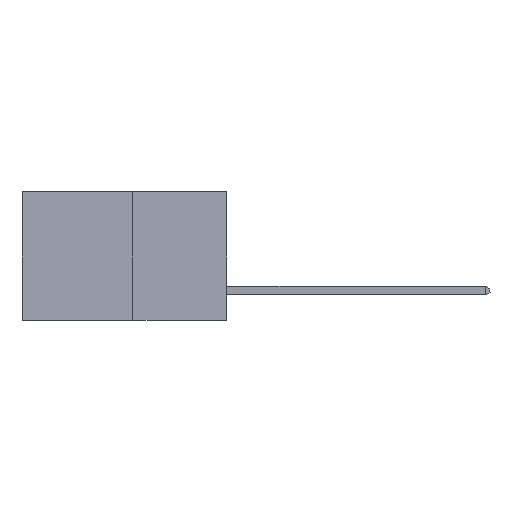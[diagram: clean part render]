
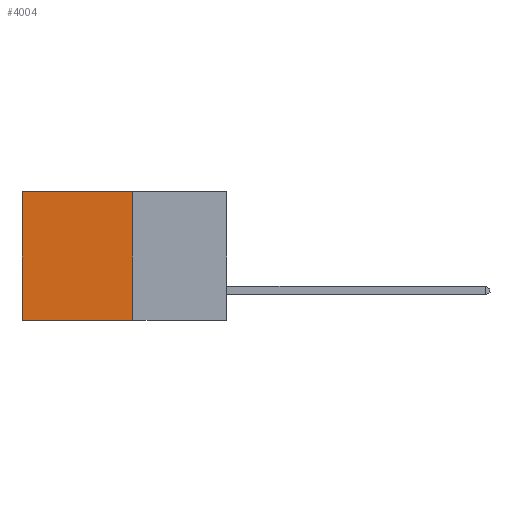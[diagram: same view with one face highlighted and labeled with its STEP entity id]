
A CAD part, left-side view. The second image highlights one B-rep face of the part: STEP entity #4004.
In plain terms, the highlighted planar face has unit normal (-1, 0, 0).
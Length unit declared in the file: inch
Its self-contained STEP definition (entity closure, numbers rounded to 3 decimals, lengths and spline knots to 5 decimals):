
#197 = VERTEX_POINT ( 'NONE', #446 ) ;
#411 = PLANE ( 'NONE',  #13152 ) ;
#446 = CARTESIAN_POINT ( 'NONE',  ( 0.277, 0.59, 0. ) ) ;
#550 = EDGE_CURVE ( 'NONE', #197, #4787, #12635, .T. ) ;
#1785 = CARTESIAN_POINT ( 'NONE',  ( 0.277, 0.27, -0.37 ) ) ;
#1812 = VERTEX_POINT ( 'NONE', #7216 ) ;
#1814 = LINE ( 'NONE', #14113, #13857 ) ;
#2046 = LINE ( 'NONE', #7939, #11106 ) ;
#2380 = DIRECTION ( 'NONE',  ( 0., 1., 0. ) ) ;
#3654 = CARTESIAN_POINT ( 'NONE',  ( 0.277, 0.27, -0.37 ) ) ;
#4004 = ADVANCED_FACE ( 'NONE', ( #12743 ), #411, .F. ) ;
#4449 = DIRECTION ( 'NONE',  ( 0., 0., -1. ) ) ;
#4787 = VERTEX_POINT ( 'NONE', #6311 ) ;
#5148 = CARTESIAN_POINT ( 'NONE',  ( 0.277, 0.59, -0.37 ) ) ;
#5973 = ORIENTED_EDGE ( 'NONE', *, *, #550, .T. ) ;
#6011 = EDGE_CURVE ( 'NONE', #1812, #7327, #2046, .T. ) ;
#6195 = VECTOR ( 'NONE', #4449, 39.37008 ) ;
#6311 = CARTESIAN_POINT ( 'NONE',  ( 0.277, 0.59, -0.37 ) ) ;
#7113 = EDGE_CURVE ( 'NONE', #1812, #197, #1814, .T. ) ;
#7196 = LINE ( 'NONE', #3654, #9926 ) ;
#7216 = CARTESIAN_POINT ( 'NONE',  ( 0.277, 0.27, 0. ) ) ;
#7327 = VERTEX_POINT ( 'NONE', #7451 ) ;
#7451 = CARTESIAN_POINT ( 'NONE',  ( 0.277, 0.27, -0.37 ) ) ;
#7939 = CARTESIAN_POINT ( 'NONE',  ( 0.277, 0.27, -0.37 ) ) ;
#7962 = DIRECTION ( 'NONE',  ( 0., 0., -1. ) ) ;
#7974 = DIRECTION ( 'NONE',  ( 1., 0., 0. ) ) ;
#8414 = EDGE_LOOP ( 'NONE', ( #5973, #9049, #12080, #15001 ) ) ;
#9049 = ORIENTED_EDGE ( 'NONE', *, *, #13432, .F. ) ;
#9926 = VECTOR ( 'NONE', #2380, 39.37008 ) ;
#11106 = VECTOR ( 'NONE', #14881, 39.37008 ) ;
#12080 = ORIENTED_EDGE ( 'NONE', *, *, #6011, .F. ) ;
#12635 = LINE ( 'NONE', #5148, #6195 ) ;
#12743 = FACE_OUTER_BOUND ( 'NONE', #8414, .T. ) ;
#13152 = AXIS2_PLACEMENT_3D ( 'NONE', #1785, #7974, #7962 ) ;
#13432 = EDGE_CURVE ( 'NONE', #7327, #4787, #7196, .T. ) ;
#13540 = DIRECTION ( 'NONE',  ( 0., 1., 0. ) ) ;
#13857 = VECTOR ( 'NONE', #13540, 39.37008 ) ;
#14113 = CARTESIAN_POINT ( 'NONE',  ( 0.277, 0.27, 0. ) ) ;
#14881 = DIRECTION ( 'NONE',  ( 0., 0., -1. ) ) ;
#15001 = ORIENTED_EDGE ( 'NONE', *, *, #7113, .T. ) ;
